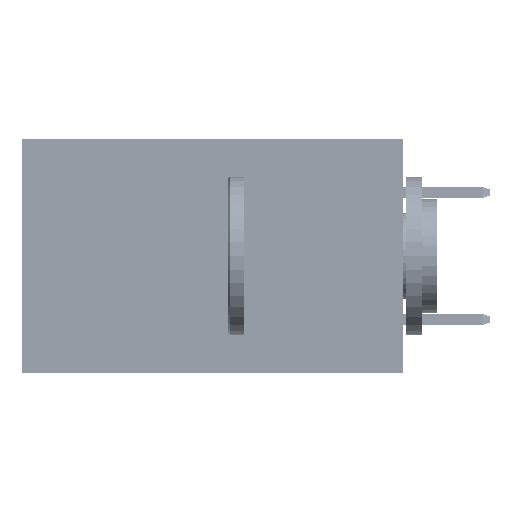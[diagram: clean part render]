
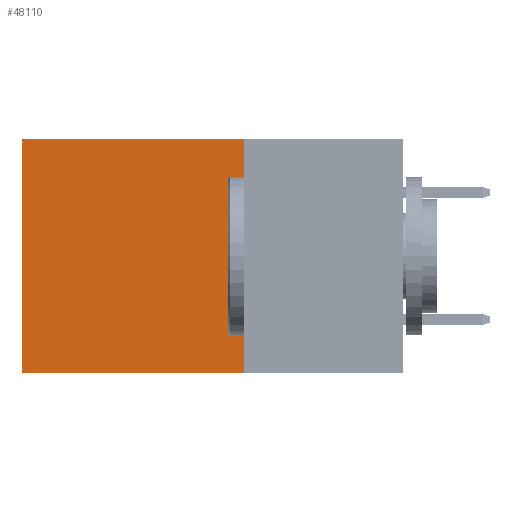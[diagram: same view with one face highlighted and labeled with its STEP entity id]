
A CAD part, left-side view. The second image highlights one B-rep face of the part: STEP entity #48110.
In plain terms, the highlighted planar face has unit normal (-1, 0, 0).
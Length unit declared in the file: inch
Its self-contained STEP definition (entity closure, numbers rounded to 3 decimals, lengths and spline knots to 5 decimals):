
#127 = DIRECTION ( 'NONE',  ( 0., 1., 0. ) ) ;
#974 = ORIENTED_EDGE ( 'NONE', *, *, #4039, .T. ) ;
#1072 = CARTESIAN_POINT ( 'NONE',  ( 0.2875, 0.25, -0.37 ) ) ;
#3688 = FACE_OUTER_BOUND ( 'NONE', #34151, .T. ) ;
#3731 = ORIENTED_EDGE ( 'NONE', *, *, #11763, .F. ) ;
#4039 = EDGE_CURVE ( 'NONE', #24827, #35609, #5455, .T. ) ;
#4241 = VECTOR ( 'NONE', #127, 39.37008 ) ;
#5455 = LINE ( 'NONE', #20007, #16564 ) ;
#5871 = EDGE_CURVE ( 'NONE', #33216, #24827, #8959, .T. ) ;
#7144 = DIRECTION ( 'NONE',  ( 0., 0., -1. ) ) ;
#8666 = DIRECTION ( 'NONE',  ( 0., 0., -1. ) ) ;
#8959 = LINE ( 'NONE', #16852, #30648 ) ;
#11763 = EDGE_CURVE ( 'NONE', #33216, #23430, #22545, .T. ) ;
#14305 = CARTESIAN_POINT ( 'NONE',  ( 0.2875, 0.6, -0.37 ) ) ;
#16564 = VECTOR ( 'NONE', #8666, 39.37008 ) ;
#16852 = CARTESIAN_POINT ( 'NONE',  ( 0.2875, 0.25, 0. ) ) ;
#17632 = CARTESIAN_POINT ( 'NONE',  ( 0.2875, 0.6, 0. ) ) ;
#20007 = CARTESIAN_POINT ( 'NONE',  ( 0.2875, 0.6, 0. ) ) ;
#22414 = CARTESIAN_POINT ( 'NONE',  ( 0.2875, 0.25, 0. ) ) ;
#22545 = LINE ( 'NONE', #44703, #34719 ) ;
#23430 = VERTEX_POINT ( 'NONE', #33379 ) ;
#24827 = VERTEX_POINT ( 'NONE', #17632 ) ;
#27899 = ORIENTED_EDGE ( 'NONE', *, *, #5871, .T. ) ;
#30648 = VECTOR ( 'NONE', #42465, 39.37008 ) ;
#33216 = VERTEX_POINT ( 'NONE', #46488 ) ;
#33249 = AXIS2_PLACEMENT_3D ( 'NONE', #22414, #34492, #7144 ) ;
#33379 = CARTESIAN_POINT ( 'NONE',  ( 0.2875, 0.25, -0.37 ) ) ;
#33466 = EDGE_CURVE ( 'NONE', #23430, #35609, #33890, .T. ) ;
#33647 = DIRECTION ( 'NONE',  ( 0., 0., -1. ) ) ;
#33890 = LINE ( 'NONE', #1072, #4241 ) ;
#34151 = EDGE_LOOP ( 'NONE', ( #974, #39657, #3731, #27899 ) ) ;
#34492 = DIRECTION ( 'NONE',  ( 1., 0., 0. ) ) ;
#34719 = VECTOR ( 'NONE', #33647, 39.37008 ) ;
#35609 = VERTEX_POINT ( 'NONE', #14305 ) ;
#37949 = PLANE ( 'NONE',  #33249 ) ;
#39657 = ORIENTED_EDGE ( 'NONE', *, *, #33466, .F. ) ;
#42465 = DIRECTION ( 'NONE',  ( 0., 1., 0. ) ) ;
#44703 = CARTESIAN_POINT ( 'NONE',  ( 0.2875, 0.25, 0. ) ) ;
#46488 = CARTESIAN_POINT ( 'NONE',  ( 0.2875, 0.25, 0. ) ) ;
#48110 = ADVANCED_FACE ( 'NONE', ( #3688 ), #37949, .F. ) ;
